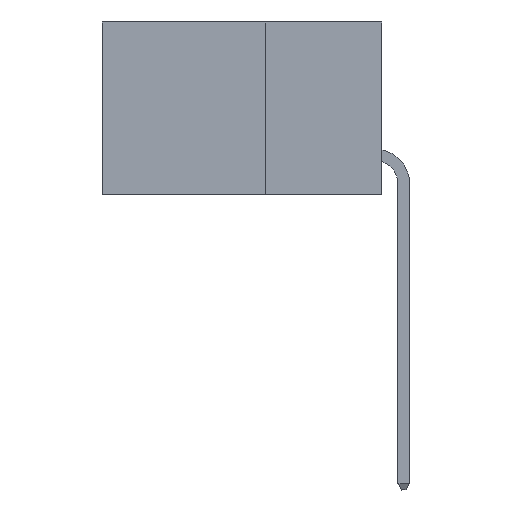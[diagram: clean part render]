
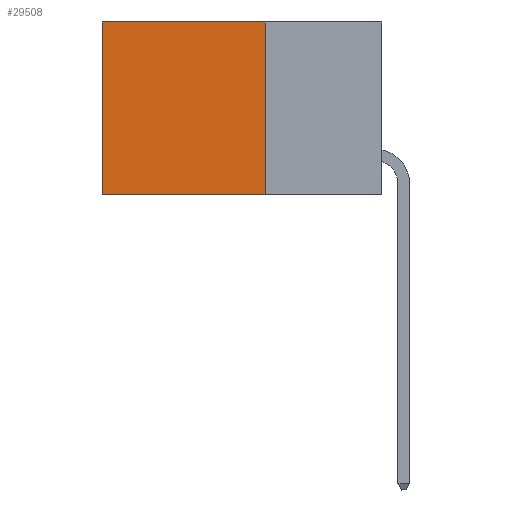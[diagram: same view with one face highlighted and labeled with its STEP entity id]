
A CAD part, left-side view. The second image highlights one B-rep face of the part: STEP entity #29508.
In plain terms, the highlighted planar face has unit normal (-1, 0, 0).
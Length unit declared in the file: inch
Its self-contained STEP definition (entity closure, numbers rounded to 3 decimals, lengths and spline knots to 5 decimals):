
#1121 = ORIENTED_EDGE ( 'NONE', *, *, #8929, .F. ) ;
#1248 = EDGE_LOOP ( 'NONE', ( #29034, #4437, #1121, #30750 ) ) ;
#1544 = CARTESIAN_POINT ( 'NONE',  ( 0.2875, 0.25, 0. ) ) ;
#3445 = PLANE ( 'NONE',  #11482 ) ;
#3920 = EDGE_CURVE ( 'NONE', #5858, #6504, #12903, .T. ) ;
#4437 = ORIENTED_EDGE ( 'NONE', *, *, #28009, .F. ) ;
#5858 = VERTEX_POINT ( 'NONE', #29090 ) ;
#6482 = FACE_OUTER_BOUND ( 'NONE', #1248, .T. ) ;
#6504 = VERTEX_POINT ( 'NONE', #14514 ) ;
#6907 = CARTESIAN_POINT ( 'NONE',  ( 0.2875, 0.25, -0.37 ) ) ;
#6949 = CARTESIAN_POINT ( 'NONE',  ( 0.2875, 0.6, 0. ) ) ;
#7358 = DIRECTION ( 'NONE',  ( 0., 1., 0. ) ) ;
#8929 = EDGE_CURVE ( 'NONE', #5858, #18396, #29015, .T. ) ;
#10431 = DIRECTION ( 'NONE',  ( 0., 1., 0. ) ) ;
#10814 = CARTESIAN_POINT ( 'NONE',  ( 0.2875, 0.25, 0. ) ) ;
#10871 = EDGE_CURVE ( 'NONE', #6504, #17201, #27006, .T. ) ;
#10924 = DIRECTION ( 'NONE',  ( 0., 0., -1. ) ) ;
#11225 = VECTOR ( 'NONE', #7358, 39.37008 ) ;
#11482 = AXIS2_PLACEMENT_3D ( 'NONE', #10814, #27885, #10924 ) ;
#11903 = DIRECTION ( 'NONE',  ( 0., 0., -1. ) ) ;
#12903 = LINE ( 'NONE', #20152, #25456 ) ;
#14514 = CARTESIAN_POINT ( 'NONE',  ( 0.2875, 0.6, 0. ) ) ;
#17201 = VERTEX_POINT ( 'NONE', #20612 ) ;
#18396 = VERTEX_POINT ( 'NONE', #6907 ) ;
#18952 = DIRECTION ( 'NONE',  ( 0., 0., -1. ) ) ;
#20152 = CARTESIAN_POINT ( 'NONE',  ( 0.2875, 0.25, 0. ) ) ;
#20612 = CARTESIAN_POINT ( 'NONE',  ( 0.2875, 0.6, -0.37 ) ) ;
#21807 = CARTESIAN_POINT ( 'NONE',  ( 0.2875, 0.25, -0.37 ) ) ;
#25456 = VECTOR ( 'NONE', #10431, 39.37008 ) ;
#25487 = VECTOR ( 'NONE', #11903, 39.37008 ) ;
#25720 = LINE ( 'NONE', #21807, #11225 ) ;
#26394 = VECTOR ( 'NONE', #18952, 39.37008 ) ;
#27006 = LINE ( 'NONE', #6949, #25487 ) ;
#27885 = DIRECTION ( 'NONE',  ( 1., 0., 0. ) ) ;
#28009 = EDGE_CURVE ( 'NONE', #18396, #17201, #25720, .T. ) ;
#29015 = LINE ( 'NONE', #1544, #26394 ) ;
#29034 = ORIENTED_EDGE ( 'NONE', *, *, #10871, .T. ) ;
#29090 = CARTESIAN_POINT ( 'NONE',  ( 0.2875, 0.25, 0. ) ) ;
#29508 = ADVANCED_FACE ( 'NONE', ( #6482 ), #3445, .F. ) ;
#30750 = ORIENTED_EDGE ( 'NONE', *, *, #3920, .T. ) ;
